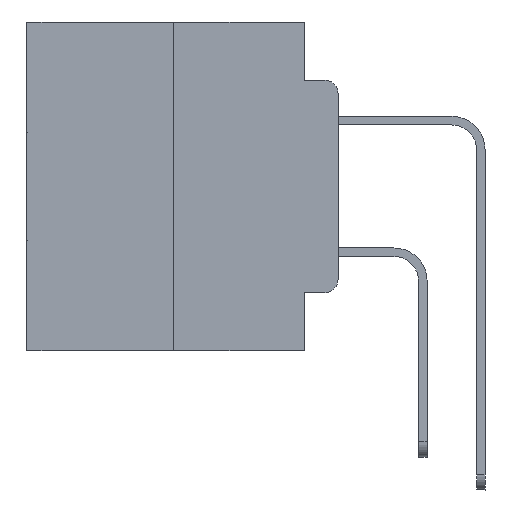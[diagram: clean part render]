
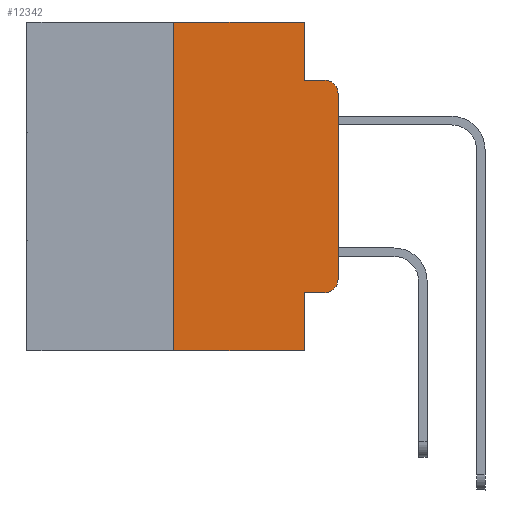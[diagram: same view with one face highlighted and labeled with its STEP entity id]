
A CAD part, left-side view. The second image highlights one B-rep face of the part: STEP entity #12342.
In plain terms, the highlighted planar face has unit normal (-1, 0, 0).
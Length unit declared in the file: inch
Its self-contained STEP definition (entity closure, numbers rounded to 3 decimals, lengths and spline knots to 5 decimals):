
#464 = CARTESIAN_POINT ( 'NONE',  ( 0., 0.02, -0.3915 ) ) ;
#688 = CARTESIAN_POINT ( 'NONE',  ( 0., 0.051, -0.4115 ) ) ;
#866 = LINE ( 'NONE', #17749, #23662 ) ;
#894 = CARTESIAN_POINT ( 'NONE',  ( 0., 0.25, -0.5 ) ) ;
#2601 = CARTESIAN_POINT ( 'NONE',  ( 0., 0., 0. ) ) ;
#3053 = VECTOR ( 'NONE', #22780, 39.37008 ) ;
#3508 = LINE ( 'NONE', #13026, #25531 ) ;
#4121 = VECTOR ( 'NONE', #5724, 39.37008 ) ;
#4223 = ORIENTED_EDGE ( 'NONE', *, *, #7095, .F. ) ;
#4513 = VERTEX_POINT ( 'NONE', #16936 ) ;
#5057 = EDGE_CURVE ( 'NONE', #23626, #17871, #8620, .T. ) ;
#5724 = DIRECTION ( 'NONE',  ( 0., -1., 0. ) ) ;
#5854 = DIRECTION ( 'NONE',  ( 0., 0., -1. ) ) ;
#5996 = EDGE_CURVE ( 'NONE', #28757, #15626, #8085, .T. ) ;
#6591 = EDGE_CURVE ( 'NONE', #11064, #4513, #14126, .T. ) ;
#6678 = DIRECTION ( 'NONE',  ( 0., -1., 0. ) ) ;
#7000 = EDGE_LOOP ( 'NONE', ( #16895, #8613, #17482, #17413, #17721, #19832, #17242, #4223, #19208, #14474 ) ) ;
#7095 = EDGE_CURVE ( 'NONE', #23626, #23935, #866, .T. ) ;
#7559 = CARTESIAN_POINT ( 'NONE',  ( 0., 0.051, -0.0885 ) ) ;
#8085 = LINE ( 'NONE', #10110, #4121 ) ;
#8613 = ORIENTED_EDGE ( 'NONE', *, *, #6591, .T. ) ;
#8620 = LINE ( 'NONE', #22631, #3053 ) ;
#9098 = DIRECTION ( 'NONE',  ( 0., 0., -1. ) ) ;
#9251 = CARTESIAN_POINT ( 'NONE',  ( 0., 0.473, 0. ) ) ;
#9698 = DIRECTION ( 'NONE',  ( -1., 0., 0. ) ) ;
#10076 = DIRECTION ( 'NONE',  ( 0., 0., -1. ) ) ;
#10110 = CARTESIAN_POINT ( 'NONE',  ( 0., 0.473, 0. ) ) ;
#11064 = VERTEX_POINT ( 'NONE', #24107 ) ;
#11200 = EDGE_CURVE ( 'NONE', #15626, #22412, #3508, .T. ) ;
#12342 = ADVANCED_FACE ( 'NONE', ( #30425 ), #27800, .F. ) ;
#13026 = CARTESIAN_POINT ( 'NONE',  ( 0., 0.051, 0. ) ) ;
#13298 = CARTESIAN_POINT ( 'NONE',  ( 0., 0.473, -0.5 ) ) ;
#13356 = EDGE_CURVE ( 'NONE', #19664, #11064, #28498, .T. ) ;
#13610 = DIRECTION ( 'NONE',  ( 1., 0., 0. ) ) ;
#13943 = AXIS2_PLACEMENT_3D ( 'NONE', #9251, #13610, #9098 ) ;
#14126 = CIRCLE ( 'NONE', #18127, 0.02 ) ;
#14474 = ORIENTED_EDGE ( 'NONE', *, *, #19896, .T. ) ;
#14483 = AXIS2_PLACEMENT_3D ( 'NONE', #464, #9698, #21387 ) ;
#15626 = VERTEX_POINT ( 'NONE', #21521 ) ;
#15940 = CARTESIAN_POINT ( 'NONE',  ( 0., 0.25, 0. ) ) ;
#16895 = ORIENTED_EDGE ( 'NONE', *, *, #13356, .T. ) ;
#16908 = VECTOR ( 'NONE', #27766, 39.37008 ) ;
#16936 = CARTESIAN_POINT ( 'NONE',  ( 0., 0.02, -0.0885 ) ) ;
#17186 = DIRECTION ( 'NONE',  ( 0., 0., -1. ) ) ;
#17242 = ORIENTED_EDGE ( 'NONE', *, *, #20656, .T. ) ;
#17413 = ORIENTED_EDGE ( 'NONE', *, *, #11200, .F. ) ;
#17482 = ORIENTED_EDGE ( 'NONE', *, *, #30245, .F. ) ;
#17721 = ORIENTED_EDGE ( 'NONE', *, *, #5996, .F. ) ;
#17749 = CARTESIAN_POINT ( 'NONE',  ( 0., 0.051, 0. ) ) ;
#17871 = VERTEX_POINT ( 'NONE', #25997 ) ;
#18127 = AXIS2_PLACEMENT_3D ( 'NONE', #21989, #21828, #17186 ) ;
#18534 = EDGE_CURVE ( 'NONE', #28688, #28757, #18730, .T. ) ;
#18730 = LINE ( 'NONE', #15940, #16908 ) ;
#18994 = DIRECTION ( 'NONE',  ( 0., 0., 1. ) ) ;
#19208 = ORIENTED_EDGE ( 'NONE', *, *, #5057, .T. ) ;
#19664 = VERTEX_POINT ( 'NONE', #28296 ) ;
#19832 = ORIENTED_EDGE ( 'NONE', *, *, #18534, .F. ) ;
#19896 = EDGE_CURVE ( 'NONE', #17871, #19664, #20435, .T. ) ;
#19968 = VECTOR ( 'NONE', #20779, 39.37008 ) ;
#20435 = CIRCLE ( 'NONE', #14483, 0.02 ) ;
#20656 = EDGE_CURVE ( 'NONE', #28688, #23935, #27957, .T. ) ;
#20779 = DIRECTION ( 'NONE',  ( 0., -1., 0. ) ) ;
#21387 = DIRECTION ( 'NONE',  ( 0., 0., -1. ) ) ;
#21521 = CARTESIAN_POINT ( 'NONE',  ( 0., 0.051, 0. ) ) ;
#21828 = DIRECTION ( 'NONE',  ( -1., 0., 0. ) ) ;
#21989 = CARTESIAN_POINT ( 'NONE',  ( 0., 0.02, -0.1085 ) ) ;
#22358 = VECTOR ( 'NONE', #18994, 39.37008 ) ;
#22412 = VERTEX_POINT ( 'NONE', #7559 ) ;
#22631 = CARTESIAN_POINT ( 'NONE',  ( 0., 0.051, -0.4115 ) ) ;
#22780 = DIRECTION ( 'NONE',  ( 0., -1., 0. ) ) ;
#23626 = VERTEX_POINT ( 'NONE', #688 ) ;
#23662 = VECTOR ( 'NONE', #5854, 39.37008 ) ;
#23793 = LINE ( 'NONE', #25839, #29337 ) ;
#23935 = VERTEX_POINT ( 'NONE', #30748 ) ;
#24107 = CARTESIAN_POINT ( 'NONE',  ( 0., 0., -0.1085 ) ) ;
#25531 = VECTOR ( 'NONE', #10076, 39.37008 ) ;
#25839 = CARTESIAN_POINT ( 'NONE',  ( 0., 0.051, -0.0885 ) ) ;
#25997 = CARTESIAN_POINT ( 'NONE',  ( 0., 0.02, -0.4115 ) ) ;
#27766 = DIRECTION ( 'NONE',  ( 0., 0., 1. ) ) ;
#27800 = PLANE ( 'NONE',  #13943 ) ;
#27957 = LINE ( 'NONE', #13298, #19968 ) ;
#28296 = CARTESIAN_POINT ( 'NONE',  ( 0., 0., -0.3915 ) ) ;
#28498 = LINE ( 'NONE', #2601, #22358 ) ;
#28675 = CARTESIAN_POINT ( 'NONE',  ( 0., 0.25, 0. ) ) ;
#28688 = VERTEX_POINT ( 'NONE', #894 ) ;
#28757 = VERTEX_POINT ( 'NONE', #28675 ) ;
#29337 = VECTOR ( 'NONE', #6678, 39.37008 ) ;
#30245 = EDGE_CURVE ( 'NONE', #22412, #4513, #23793, .T. ) ;
#30425 = FACE_OUTER_BOUND ( 'NONE', #7000, .T. ) ;
#30748 = CARTESIAN_POINT ( 'NONE',  ( 0., 0.051, -0.5 ) ) ;
